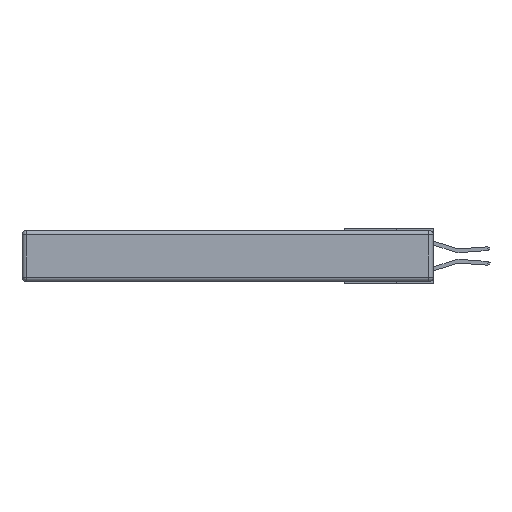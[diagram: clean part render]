
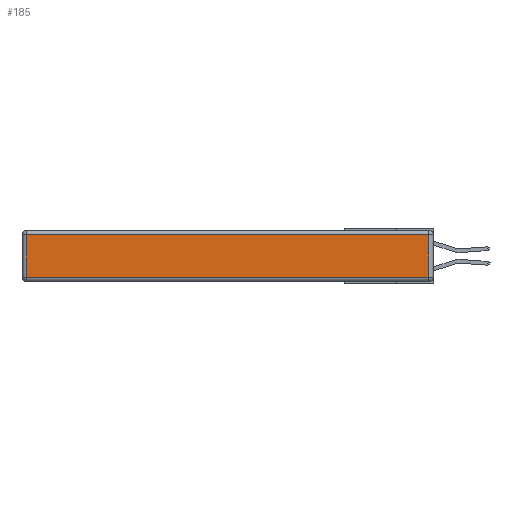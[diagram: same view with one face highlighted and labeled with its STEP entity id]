
A CAD part, left-side view. The second image highlights one B-rep face of the part: STEP entity #185.
In plain terms, the highlighted planar face has unit normal (-1, 0, 0).
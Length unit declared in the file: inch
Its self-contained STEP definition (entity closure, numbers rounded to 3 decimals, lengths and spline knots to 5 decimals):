
#185 = ADVANCED_FACE ( 'NONE', ( #9895 ), #13162, .T. ) ;
#685 = CARTESIAN_POINT ( 'NONE',  ( 0., 2.72, -0.03 ) ) ;
#797 = ORIENTED_EDGE ( 'NONE', *, *, #2888, .T. ) ;
#929 = DIRECTION ( 'NONE',  ( 0., 0., -1. ) ) ;
#985 = CARTESIAN_POINT ( 'NONE',  ( 0., 2.72, -0.343 ) ) ;
#2298 = AXIS2_PLACEMENT_3D ( 'NONE', #6310, #5117, #13065 ) ;
#2794 = VERTEX_POINT ( 'NONE', #8399 ) ;
#2807 = DIRECTION ( 'NONE',  ( 0., -1., 0. ) ) ;
#2833 = DIRECTION ( 'NONE',  ( 0., 0., 1. ) ) ;
#2888 = EDGE_CURVE ( 'NONE', #6680, #4447, #10355, .T. ) ;
#3115 = LINE ( 'NONE', #10134, #3831 ) ;
#3631 = CARTESIAN_POINT ( 'NONE',  ( 0., 0.03, -0.313 ) ) ;
#3831 = VECTOR ( 'NONE', #12417, 39.37008 ) ;
#4097 = ORIENTED_EDGE ( 'NONE', *, *, #9402, .T. ) ;
#4447 = VERTEX_POINT ( 'NONE', #9855 ) ;
#5117 = DIRECTION ( 'NONE',  ( -1., 0., 0. ) ) ;
#5787 = ORIENTED_EDGE ( 'NONE', *, *, #7176, .T. ) ;
#6310 = CARTESIAN_POINT ( 'NONE',  ( 0., 0., -0.343 ) ) ;
#6680 = VERTEX_POINT ( 'NONE', #3631 ) ;
#7176 = EDGE_CURVE ( 'NONE', #4447, #10223, #3115, .T. ) ;
#7318 = VECTOR ( 'NONE', #2833, 39.37008 ) ;
#8399 = CARTESIAN_POINT ( 'NONE',  ( 0., 2.72, -0.313 ) ) ;
#9402 = EDGE_CURVE ( 'NONE', #2794, #6680, #13891, .T. ) ;
#9413 = LINE ( 'NONE', #985, #13859 ) ;
#9855 = CARTESIAN_POINT ( 'NONE',  ( 0., 0.03, -0.03 ) ) ;
#9895 = FACE_OUTER_BOUND ( 'NONE', #11807, .T. ) ;
#10134 = CARTESIAN_POINT ( 'NONE',  ( 0., 2.75, -0.03 ) ) ;
#10223 = VERTEX_POINT ( 'NONE', #685 ) ;
#10355 = LINE ( 'NONE', #13019, #7318 ) ;
#11092 = ORIENTED_EDGE ( 'NONE', *, *, #12238, .T. ) ;
#11094 = VECTOR ( 'NONE', #2807, 39.37008 ) ;
#11807 = EDGE_LOOP ( 'NONE', ( #4097, #797, #5787, #11092 ) ) ;
#12060 = CARTESIAN_POINT ( 'NONE',  ( 0., 0., -0.313 ) ) ;
#12238 = EDGE_CURVE ( 'NONE', #10223, #2794, #9413, .T. ) ;
#12417 = DIRECTION ( 'NONE',  ( 0., 1., 0. ) ) ;
#13019 = CARTESIAN_POINT ( 'NONE',  ( 0., 0.03, -0.343 ) ) ;
#13065 = DIRECTION ( 'NONE',  ( 0., 0., 1. ) ) ;
#13162 = PLANE ( 'NONE',  #2298 ) ;
#13859 = VECTOR ( 'NONE', #929, 39.37008 ) ;
#13891 = LINE ( 'NONE', #12060, #11094 ) ;
